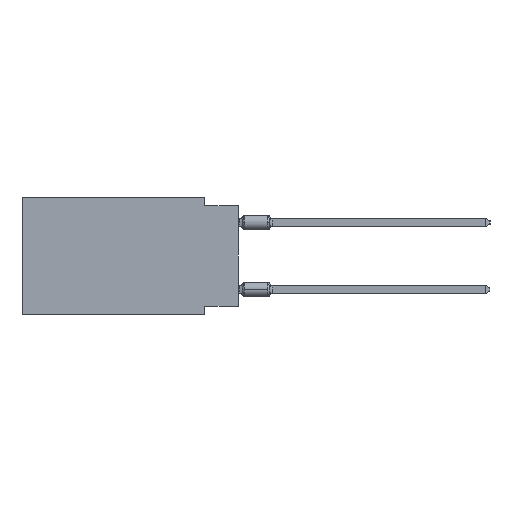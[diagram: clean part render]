
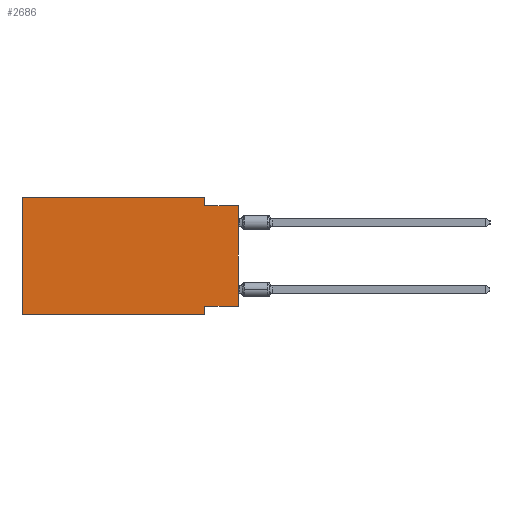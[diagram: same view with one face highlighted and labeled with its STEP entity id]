
A CAD part, left-side view. The second image highlights one B-rep face of the part: STEP entity #2686.
In plain terms, the highlighted planar face has unit normal (-1, 0, 0).
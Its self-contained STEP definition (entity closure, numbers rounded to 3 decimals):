
#1161 = VECTOR ( 'NONE', #45476, 1000. ) ;
#2686 = ADVANCED_FACE ( 'NONE', ( #20603 ), #12237, .F. ) ;
#2877 = DIRECTION ( 'NONE',  ( 0., 0., 1. ) ) ;
#3183 = ORIENTED_EDGE ( 'NONE', *, *, #39805, .F. ) ;
#7911 = ORIENTED_EDGE ( 'NONE', *, *, #39015, .F. ) ;
#8396 = ORIENTED_EDGE ( 'NONE', *, *, #44697, .F. ) ;
#8463 = CARTESIAN_POINT ( 'NONE',  ( 0., 2.54, -0.635 ) ) ;
#8717 = CARTESIAN_POINT ( 'NONE',  ( 0., 0., -0.635 ) ) ;
#9080 = EDGE_CURVE ( 'NONE', #51517, #24697, #18523, .T. ) ;
#9546 = DIRECTION ( 'NONE',  ( 0., -1., 0. ) ) ;
#10574 = VERTEX_POINT ( 'NONE', #8717 ) ;
#11026 = EDGE_CURVE ( 'NONE', #24330, #10574, #25570, .T. ) ;
#11228 = LINE ( 'NONE', #39669, #46884 ) ;
#11345 = ORIENTED_EDGE ( 'NONE', *, *, #42779, .F. ) ;
#12165 = CARTESIAN_POINT ( 'NONE',  ( 0., 2.54, -8.89 ) ) ;
#12237 = PLANE ( 'NONE',  #27012 ) ;
#13314 = LINE ( 'NONE', #13583, #25043 ) ;
#13583 = CARTESIAN_POINT ( 'NONE',  ( 0., 16.383, 0. ) ) ;
#14850 = LINE ( 'NONE', #36031, #29787 ) ;
#14856 = CARTESIAN_POINT ( 'NONE',  ( 0., 2.54, 0. ) ) ;
#16660 = EDGE_CURVE ( 'NONE', #35918, #10574, #11228, .T. ) ;
#17017 = LINE ( 'NONE', #45197, #51741 ) ;
#18523 = LINE ( 'NONE', #34877, #52223 ) ;
#19959 = CARTESIAN_POINT ( 'NONE',  ( 0., 2.54, -8.255 ) ) ;
#20420 = VERTEX_POINT ( 'NONE', #19959 ) ;
#20603 = FACE_OUTER_BOUND ( 'NONE', #40598, .T. ) ;
#24330 = VERTEX_POINT ( 'NONE', #8463 ) ;
#24612 = CARTESIAN_POINT ( 'NONE',  ( 0., 16.383, 0. ) ) ;
#24697 = VERTEX_POINT ( 'NONE', #12165 ) ;
#24978 = ORIENTED_EDGE ( 'NONE', *, *, #9080, .T. ) ;
#25043 = VECTOR ( 'NONE', #9546, 1000. ) ;
#25570 = LINE ( 'NONE', #45161, #47265 ) ;
#27012 = AXIS2_PLACEMENT_3D ( 'NONE', #24612, #36387, #49530 ) ;
#27207 = DIRECTION ( 'NONE',  ( 0., 0., -1. ) ) ;
#28520 = VERTEX_POINT ( 'NONE', #14856 ) ;
#28987 = ORIENTED_EDGE ( 'NONE', *, *, #11026, .F. ) ;
#29136 = LINE ( 'NONE', #37412, #1161 ) ;
#29787 = VECTOR ( 'NONE', #27207, 1000. ) ;
#30437 = CARTESIAN_POINT ( 'NONE',  ( 0., 16.383, -8.89 ) ) ;
#30463 = EDGE_CURVE ( 'NONE', #20420, #24697, #14850, .T. ) ;
#33085 = DIRECTION ( 'NONE',  ( 0., -1., 0. ) ) ;
#33900 = CARTESIAN_POINT ( 'NONE',  ( 0., 0., -8.255 ) ) ;
#34233 = ORIENTED_EDGE ( 'NONE', *, *, #30463, .F. ) ;
#34877 = CARTESIAN_POINT ( 'NONE',  ( 0., 16.383, -8.89 ) ) ;
#35350 = CARTESIAN_POINT ( 'NONE',  ( 0., 0., -8.255 ) ) ;
#35387 = DIRECTION ( 'NONE',  ( 0., -1., 0. ) ) ;
#35918 = VERTEX_POINT ( 'NONE', #35350 ) ;
#36031 = CARTESIAN_POINT ( 'NONE',  ( 0., 2.54, -8.89 ) ) ;
#36382 = VECTOR ( 'NONE', #42223, 1000. ) ;
#36387 = DIRECTION ( 'NONE',  ( 1., 0., 0. ) ) ;
#37412 = CARTESIAN_POINT ( 'NONE',  ( 0., 16.383, 0. ) ) ;
#38311 = ORIENTED_EDGE ( 'NONE', *, *, #16660, .T. ) ;
#39015 = EDGE_CURVE ( 'NONE', #51517, #46472, #29136, .T. ) ;
#39669 = CARTESIAN_POINT ( 'NONE',  ( 0., 0., 0. ) ) ;
#39805 = EDGE_CURVE ( 'NONE', #35918, #20420, #42762, .T. ) ;
#40598 = EDGE_LOOP ( 'NONE', ( #38311, #28987, #8396, #11345, #7911, #24978, #34233, #3183 ) ) ;
#41438 = DIRECTION ( 'NONE',  ( 0., 0., -1. ) ) ;
#42223 = DIRECTION ( 'NONE',  ( 0., 1., 0. ) ) ;
#42762 = LINE ( 'NONE', #33900, #36382 ) ;
#42779 = EDGE_CURVE ( 'NONE', #46472, #28520, #13314, .T. ) ;
#44697 = EDGE_CURVE ( 'NONE', #28520, #24330, #17017, .T. ) ;
#45161 = CARTESIAN_POINT ( 'NONE',  ( 0., 0., -0.635 ) ) ;
#45197 = CARTESIAN_POINT ( 'NONE',  ( 0., 2.54, 0. ) ) ;
#45476 = DIRECTION ( 'NONE',  ( 0., 0., 1. ) ) ;
#46472 = VERTEX_POINT ( 'NONE', #48395 ) ;
#46884 = VECTOR ( 'NONE', #2877, 1000. ) ;
#47265 = VECTOR ( 'NONE', #33085, 1000. ) ;
#48395 = CARTESIAN_POINT ( 'NONE',  ( 0., 16.383, 0. ) ) ;
#49530 = DIRECTION ( 'NONE',  ( 0., 0., -1. ) ) ;
#51517 = VERTEX_POINT ( 'NONE', #30437 ) ;
#51741 = VECTOR ( 'NONE', #41438, 1000. ) ;
#52223 = VECTOR ( 'NONE', #35387, 1000. ) ;
